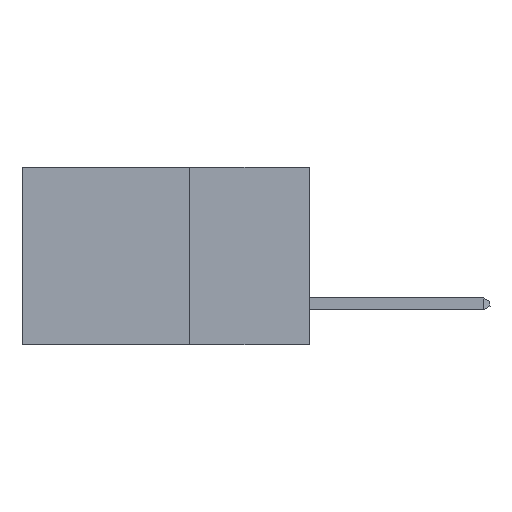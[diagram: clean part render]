
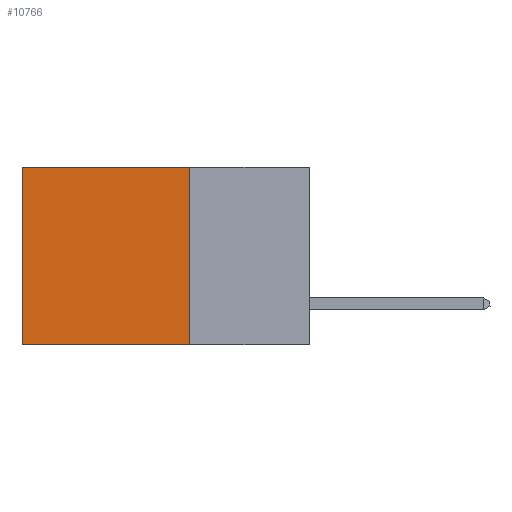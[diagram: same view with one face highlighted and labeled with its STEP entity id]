
A CAD part, left-side view. The second image highlights one B-rep face of the part: STEP entity #10766.
In plain terms, the highlighted planar face has unit normal (-1, 0, 0).
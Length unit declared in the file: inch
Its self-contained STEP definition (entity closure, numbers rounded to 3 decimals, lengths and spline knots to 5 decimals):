
#295 = ORIENTED_EDGE ( 'NONE', *, *, #5015, .F. ) ;
#363 = VECTOR ( 'NONE', #7913, 39.37008 ) ;
#583 = ORIENTED_EDGE ( 'NONE', *, *, #1616, .F. ) ;
#800 = LINE ( 'NONE', #14508, #7691 ) ;
#849 = CARTESIAN_POINT ( 'NONE',  ( 0.2875, 0.6, -0.37 ) ) ;
#956 = DIRECTION ( 'NONE',  ( 0., 1., 0. ) ) ;
#1616 = EDGE_CURVE ( 'NONE', #11899, #10538, #800, .T. ) ;
#2622 = VERTEX_POINT ( 'NONE', #849 ) ;
#2690 = CARTESIAN_POINT ( 'NONE',  ( 0.2875, 0.25, 0. ) ) ;
#2765 = VECTOR ( 'NONE', #10804, 39.37008 ) ;
#3204 = CARTESIAN_POINT ( 'NONE',  ( 0.2875, 0.25, -0.37 ) ) ;
#3422 = VERTEX_POINT ( 'NONE', #12411 ) ;
#3791 = DIRECTION ( 'NONE',  ( 1., 0., 0. ) ) ;
#4013 = ORIENTED_EDGE ( 'NONE', *, *, #13511, .T. ) ;
#4863 = VECTOR ( 'NONE', #956, 39.37008 ) ;
#5015 = EDGE_CURVE ( 'NONE', #10538, #2622, #11832, .T. ) ;
#6142 = CARTESIAN_POINT ( 'NONE',  ( 0.2875, 0.25, -0.37 ) ) ;
#6407 = AXIS2_PLACEMENT_3D ( 'NONE', #2690, #3791, #8913 ) ;
#7120 = DIRECTION ( 'NONE',  ( 0., 0., -1. ) ) ;
#7458 = LINE ( 'NONE', #8024, #363 ) ;
#7546 = PLANE ( 'NONE',  #6407 ) ;
#7691 = VECTOR ( 'NONE', #7120, 39.37008 ) ;
#7913 = DIRECTION ( 'NONE',  ( 0., 0., -1. ) ) ;
#8024 = CARTESIAN_POINT ( 'NONE',  ( 0.2875, 0.6, 0. ) ) ;
#8913 = DIRECTION ( 'NONE',  ( 0., 0., -1. ) ) ;
#10187 = LINE ( 'NONE', #12074, #2765 ) ;
#10538 = VERTEX_POINT ( 'NONE', #3204 ) ;
#10766 = ADVANCED_FACE ( 'NONE', ( #10813 ), #7546, .F. ) ;
#10804 = DIRECTION ( 'NONE',  ( 0., 1., 0. ) ) ;
#10813 = FACE_OUTER_BOUND ( 'NONE', #14267, .T. ) ;
#11832 = LINE ( 'NONE', #6142, #4863 ) ;
#11899 = VERTEX_POINT ( 'NONE', #14338 ) ;
#12074 = CARTESIAN_POINT ( 'NONE',  ( 0.2875, 0.25, 0. ) ) ;
#12411 = CARTESIAN_POINT ( 'NONE',  ( 0.2875, 0.6, 0. ) ) ;
#13511 = EDGE_CURVE ( 'NONE', #3422, #2622, #7458, .T. ) ;
#14039 = EDGE_CURVE ( 'NONE', #11899, #3422, #10187, .T. ) ;
#14267 = EDGE_LOOP ( 'NONE', ( #4013, #295, #583, #14298 ) ) ;
#14298 = ORIENTED_EDGE ( 'NONE', *, *, #14039, .T. ) ;
#14338 = CARTESIAN_POINT ( 'NONE',  ( 0.2875, 0.25, 0. ) ) ;
#14508 = CARTESIAN_POINT ( 'NONE',  ( 0.2875, 0.25, 0. ) ) ;
